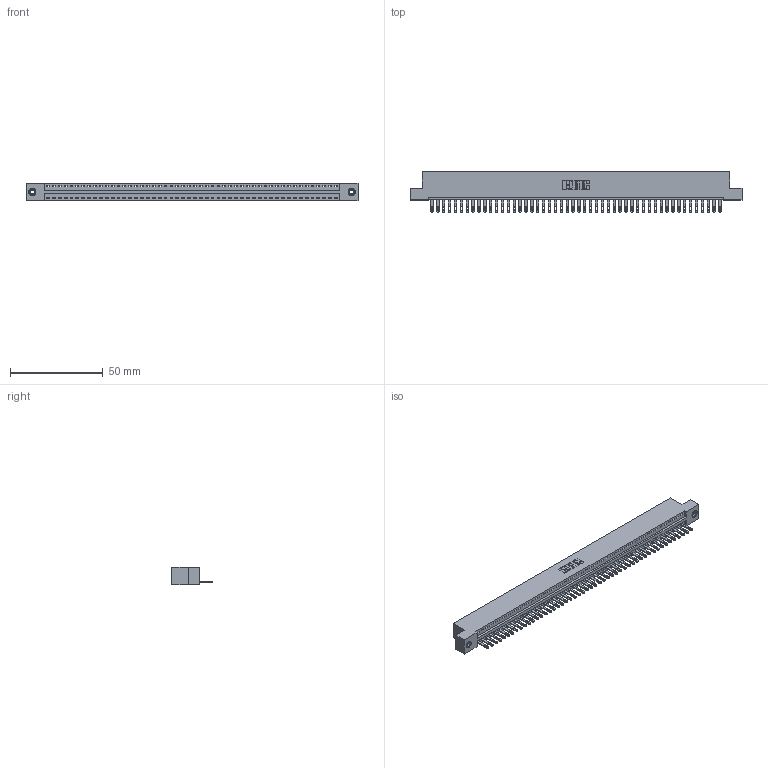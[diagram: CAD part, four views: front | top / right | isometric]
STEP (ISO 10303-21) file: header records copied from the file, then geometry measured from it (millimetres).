
FILE_DESCRIPTION (( 'STEP AP203' ), '1' );
FILE_NAME ('346-050-500-108.STEP', '2022-05-10T02:29:29', ( '' ), ( '' ), 'SwSTEP 2.0', 'SolidWorks 2020', '' );
FILE_SCHEMA (( 'CONFIG_CONTROL_DESIGN' ));
Length unit declared in the file: inch
Products named in the file (4): 345-250-001_345-250-003-102; 346 Part_Flush Mounting Lugs - 0.156 Dia-TI; 346-050-500-108; 345-292-001_345-293-100
Assembly tree (53 placements, depth 2):
  346-050-500-108
    346 Part_Flush Mounting Lugs - 0.156 Dia-TI
    345-292-001_345-293-100  x50
    345-250-001_345-250-003-102  x2
Bounding box: 179.32 x 21.84 x 9.4 mm (x, y, z)
Volume: 17244.8 mm3; surface area: 21778.4 mm2
Topology: 53 solids, 53 shells, 2882 faces, 8865 edges, 5902 vertices
Faces by surface type: plane 1808, cylinder 1058, cone 12, torus 4
Entity records: 31070 total; most frequent: CARTESIAN_POINT 5305, ORIENTED_EDGE 5282, DIRECTION 4699, EDGE_CURVE 2641, VECTOR 2285, LINE 2285, VERTEX_POINT 1756, AXIS2_PLACEMENT_3D 1207
